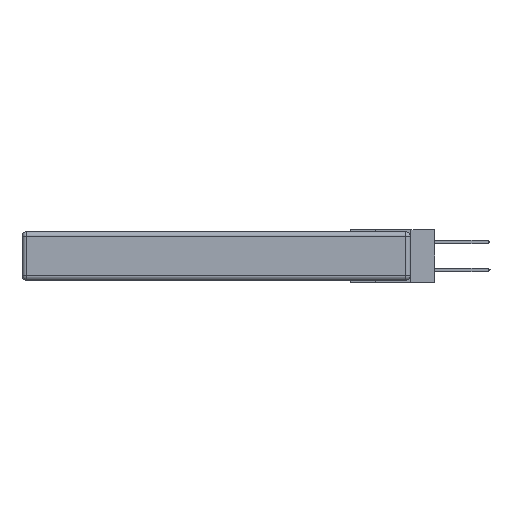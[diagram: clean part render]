
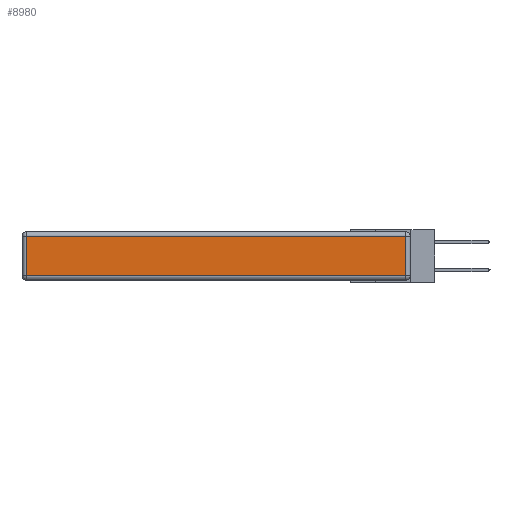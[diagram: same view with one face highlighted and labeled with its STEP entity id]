
A CAD part, left-side view. The second image highlights one B-rep face of the part: STEP entity #8980.
In plain terms, the highlighted planar face has unit normal (-1, 0, 0).
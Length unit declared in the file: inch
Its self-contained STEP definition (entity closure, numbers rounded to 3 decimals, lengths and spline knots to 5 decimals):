
#1349 = DIRECTION ( 'NONE',  ( 0., 1., 0. ) ) ;
#1580 = VECTOR ( 'NONE', #24830, 39.37008 ) ;
#1791 = EDGE_CURVE ( 'NONE', #8979, #1870, #18870, .T. ) ;
#1870 = VERTEX_POINT ( 'NONE', #4166 ) ;
#2646 = ORIENTED_EDGE ( 'NONE', *, *, #1791, .T. ) ;
#4166 = CARTESIAN_POINT ( 'NONE',  ( 0., 2.72, -0.03 ) ) ;
#4717 = VECTOR ( 'NONE', #1349, 39.37008 ) ;
#4793 = EDGE_CURVE ( 'NONE', #9926, #28819, #31413, .T. ) ;
#5091 = ORIENTED_EDGE ( 'NONE', *, *, #18253, .T. ) ;
#6051 = ORIENTED_EDGE ( 'NONE', *, *, #22806, .T. ) ;
#7544 = VECTOR ( 'NONE', #14289, 39.37008 ) ;
#8254 = DIRECTION ( 'NONE',  ( -1., 0., 0. ) ) ;
#8979 = VERTEX_POINT ( 'NONE', #20336 ) ;
#8980 = ADVANCED_FACE ( 'NONE', ( #29093 ), #22889, .T. ) ;
#9926 = VERTEX_POINT ( 'NONE', #10506 ) ;
#10506 = CARTESIAN_POINT ( 'NONE',  ( 0., 2.72, -0.313 ) ) ;
#11819 = CARTESIAN_POINT ( 'NONE',  ( 0., 2.72, -0.343 ) ) ;
#13040 = CARTESIAN_POINT ( 'NONE',  ( 0., 0., -0.343 ) ) ;
#13738 = AXIS2_PLACEMENT_3D ( 'NONE', #13040, #8254, #29826 ) ;
#13819 = CARTESIAN_POINT ( 'NONE',  ( 0., 2.75, -0.03 ) ) ;
#14289 = DIRECTION ( 'NONE',  ( 0., 0., -1. ) ) ;
#15406 = LINE ( 'NONE', #28789, #24573 ) ;
#15488 = ORIENTED_EDGE ( 'NONE', *, *, #4793, .T. ) ;
#18253 = EDGE_CURVE ( 'NONE', #28819, #8979, #15406, .T. ) ;
#18870 = LINE ( 'NONE', #13819, #4717 ) ;
#20336 = CARTESIAN_POINT ( 'NONE',  ( 0., 0.03, -0.03 ) ) ;
#22580 = CARTESIAN_POINT ( 'NONE',  ( 0., 0., -0.313 ) ) ;
#22806 = EDGE_CURVE ( 'NONE', #1870, #9926, #22872, .T. ) ;
#22872 = LINE ( 'NONE', #11819, #7544 ) ;
#22889 = PLANE ( 'NONE',  #13738 ) ;
#24573 = VECTOR ( 'NONE', #26451, 39.37008 ) ;
#24791 = CARTESIAN_POINT ( 'NONE',  ( 0., 0.03, -0.313 ) ) ;
#24830 = DIRECTION ( 'NONE',  ( 0., -1., 0. ) ) ;
#25122 = EDGE_LOOP ( 'NONE', ( #15488, #5091, #2646, #6051 ) ) ;
#26451 = DIRECTION ( 'NONE',  ( 0., 0., 1. ) ) ;
#28789 = CARTESIAN_POINT ( 'NONE',  ( 0., 0.03, -0.343 ) ) ;
#28819 = VERTEX_POINT ( 'NONE', #24791 ) ;
#29093 = FACE_OUTER_BOUND ( 'NONE', #25122, .T. ) ;
#29826 = DIRECTION ( 'NONE',  ( 0., 0., 1. ) ) ;
#31413 = LINE ( 'NONE', #22580, #1580 ) ;
